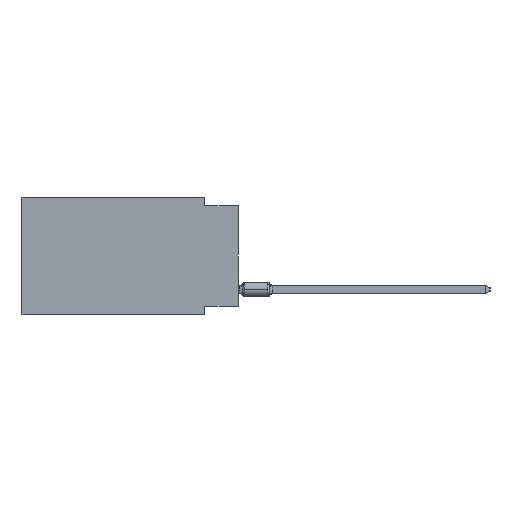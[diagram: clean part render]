
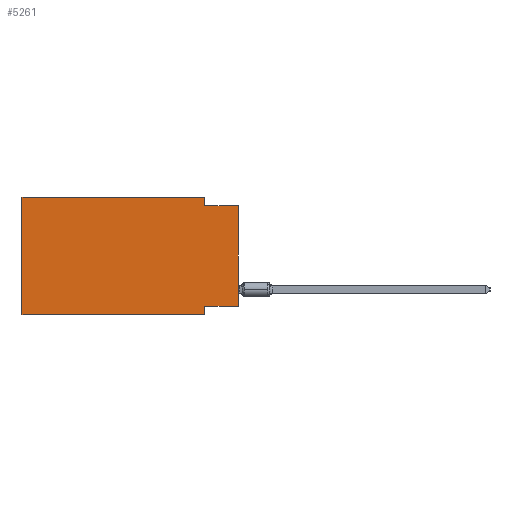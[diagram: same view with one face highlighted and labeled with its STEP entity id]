
A CAD part, left-side view. The second image highlights one B-rep face of the part: STEP entity #5261.
In plain terms, the highlighted planar face has unit normal (-1, 0, 0).
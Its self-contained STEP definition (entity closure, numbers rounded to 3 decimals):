
#198 = CARTESIAN_POINT ( 'NONE',  ( 0., 2.54, -8.89 ) ) ;
#1487 = LINE ( 'NONE', #7521, #20935 ) ;
#1491 = AXIS2_PLACEMENT_3D ( 'NONE', #10956, #23435, #36084 ) ;
#1589 = CARTESIAN_POINT ( 'NONE',  ( 0., 2.54, 0. ) ) ;
#1690 = PLANE ( 'NONE',  #1491 ) ;
#2073 = ORIENTED_EDGE ( 'NONE', *, *, #3474, .F. ) ;
#3431 = EDGE_CURVE ( 'NONE', #23852, #38159, #1487, .T. ) ;
#3474 = EDGE_CURVE ( 'NONE', #38159, #30159, #13570, .T. ) ;
#4827 = EDGE_LOOP ( 'NONE', ( #15525, #19351, #23716, #2073, #5074, #8871, #36400, #5251 ) ) ;
#5074 = ORIENTED_EDGE ( 'NONE', *, *, #3431, .F. ) ;
#5251 = ORIENTED_EDGE ( 'NONE', *, *, #27241, .F. ) ;
#5261 = ADVANCED_FACE ( 'NONE', ( #14181 ), #1690, .F. ) ;
#5477 = VECTOR ( 'NONE', #8078, 1000. ) ;
#6372 = VERTEX_POINT ( 'NONE', #16597 ) ;
#7330 = DIRECTION ( 'NONE',  ( 0., -1., 0. ) ) ;
#7521 = CARTESIAN_POINT ( 'NONE',  ( 0., 16.383, 0. ) ) ;
#7903 = VERTEX_POINT ( 'NONE', #9560 ) ;
#8078 = DIRECTION ( 'NONE',  ( 0., -1., 0. ) ) ;
#8400 = LINE ( 'NONE', #26280, #33794 ) ;
#8871 = ORIENTED_EDGE ( 'NONE', *, *, #18452, .T. ) ;
#9014 = DIRECTION ( 'NONE',  ( 0., -1., 0. ) ) ;
#9560 = CARTESIAN_POINT ( 'NONE',  ( 0., 0., -0.635 ) ) ;
#10509 = LINE ( 'NONE', #19983, #28812 ) ;
#10956 = CARTESIAN_POINT ( 'NONE',  ( 0., 16.383, 0. ) ) ;
#12095 = CARTESIAN_POINT ( 'NONE',  ( 0., 0., -8.255 ) ) ;
#13570 = LINE ( 'NONE', #31671, #16416 ) ;
#14181 = FACE_OUTER_BOUND ( 'NONE', #4827, .T. ) ;
#14445 = EDGE_CURVE ( 'NONE', #38711, #7903, #31396, .T. ) ;
#15525 = ORIENTED_EDGE ( 'NONE', *, *, #14445, .T. ) ;
#16416 = VECTOR ( 'NONE', #7330, 1000. ) ;
#16597 = CARTESIAN_POINT ( 'NONE',  ( 0., 2.54, -8.255 ) ) ;
#18121 = VERTEX_POINT ( 'NONE', #198 ) ;
#18452 = EDGE_CURVE ( 'NONE', #23852, #18121, #36552, .T. ) ;
#18697 = CARTESIAN_POINT ( 'NONE',  ( 0., 2.54, -8.89 ) ) ;
#19351 = ORIENTED_EDGE ( 'NONE', *, *, #35941, .F. ) ;
#19983 = CARTESIAN_POINT ( 'NONE',  ( 0., 0., -8.255 ) ) ;
#20404 = EDGE_CURVE ( 'NONE', #6372, #18121, #36968, .T. ) ;
#20935 = VECTOR ( 'NONE', #38078, 1000. ) ;
#20948 = CARTESIAN_POINT ( 'NONE',  ( 0., 0., -0.635 ) ) ;
#21350 = CARTESIAN_POINT ( 'NONE',  ( 0., 2.54, -0.635 ) ) ;
#22740 = CARTESIAN_POINT ( 'NONE',  ( 0., 0., 0. ) ) ;
#23435 = DIRECTION ( 'NONE',  ( 1., 0., 0. ) ) ;
#23716 = ORIENTED_EDGE ( 'NONE', *, *, #38097, .F. ) ;
#23852 = VERTEX_POINT ( 'NONE', #32645 ) ;
#25806 = VECTOR ( 'NONE', #9014, 1000. ) ;
#26280 = CARTESIAN_POINT ( 'NONE',  ( 0., 2.54, 0. ) ) ;
#27241 = EDGE_CURVE ( 'NONE', #38711, #6372, #10509, .T. ) ;
#28812 = VECTOR ( 'NONE', #35049, 1000. ) ;
#30159 = VERTEX_POINT ( 'NONE', #1589 ) ;
#31396 = LINE ( 'NONE', #22740, #34859 ) ;
#31671 = CARTESIAN_POINT ( 'NONE',  ( 0., 16.383, 0. ) ) ;
#31976 = DIRECTION ( 'NONE',  ( 0., 0., 1. ) ) ;
#32122 = DIRECTION ( 'NONE',  ( 0., 0., -1. ) ) ;
#32645 = CARTESIAN_POINT ( 'NONE',  ( 0., 16.383, -8.89 ) ) ;
#33794 = VECTOR ( 'NONE', #32122, 1000. ) ;
#34859 = VECTOR ( 'NONE', #31976, 1000. ) ;
#35049 = DIRECTION ( 'NONE',  ( 0., 1., 0. ) ) ;
#35941 = EDGE_CURVE ( 'NONE', #37453, #7903, #36032, .T. ) ;
#36032 = LINE ( 'NONE', #20948, #5477 ) ;
#36084 = DIRECTION ( 'NONE',  ( 0., 0., -1. ) ) ;
#36351 = CARTESIAN_POINT ( 'NONE',  ( 0., 16.383, -8.89 ) ) ;
#36400 = ORIENTED_EDGE ( 'NONE', *, *, #20404, .F. ) ;
#36552 = LINE ( 'NONE', #36351, #25806 ) ;
#36968 = LINE ( 'NONE', #18697, #38755 ) ;
#37453 = VERTEX_POINT ( 'NONE', #21350 ) ;
#37872 = DIRECTION ( 'NONE',  ( 0., 0., -1. ) ) ;
#38078 = DIRECTION ( 'NONE',  ( 0., 0., 1. ) ) ;
#38097 = EDGE_CURVE ( 'NONE', #30159, #37453, #8400, .T. ) ;
#38159 = VERTEX_POINT ( 'NONE', #39150 ) ;
#38711 = VERTEX_POINT ( 'NONE', #12095 ) ;
#38755 = VECTOR ( 'NONE', #37872, 1000. ) ;
#39150 = CARTESIAN_POINT ( 'NONE',  ( 0., 16.383, 0. ) ) ;
